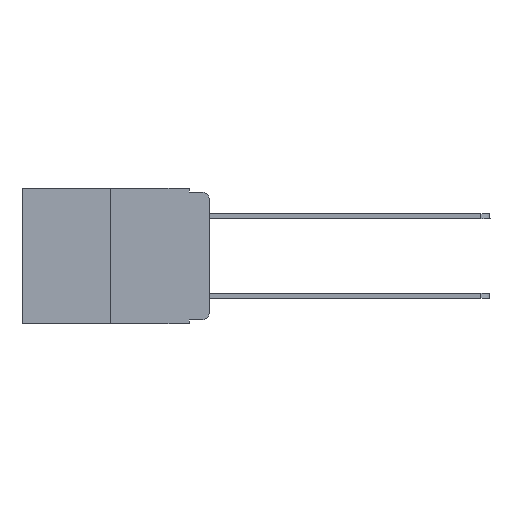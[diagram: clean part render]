
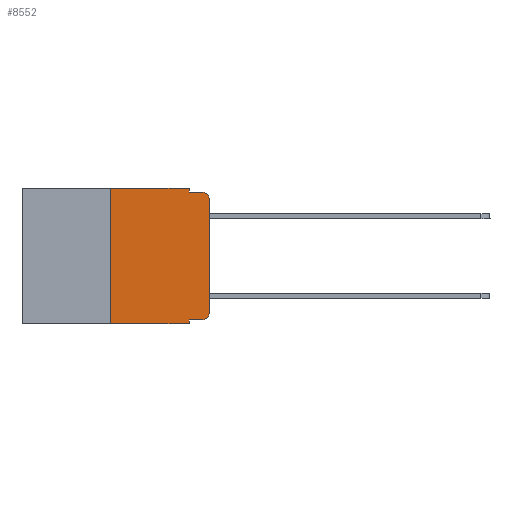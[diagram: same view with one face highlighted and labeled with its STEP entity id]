
A CAD part, left-side view. The second image highlights one B-rep face of the part: STEP entity #8552.
In plain terms, the highlighted planar face has unit normal (-1, 0, 0).
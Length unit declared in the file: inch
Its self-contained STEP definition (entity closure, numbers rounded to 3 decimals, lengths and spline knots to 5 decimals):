
#373 = VERTEX_POINT ( 'NONE', #17408 ) ;
#521 = CARTESIAN_POINT ( 'NONE',  ( 0., 0.473, 0. ) ) ;
#603 = EDGE_CURVE ( 'NONE', #18693, #10837, #5304, .T. ) ;
#614 = AXIS2_PLACEMENT_3D ( 'NONE', #3206, #13170, #5791 ) ;
#1064 = CARTESIAN_POINT ( 'NONE',  ( 0., 0.051, -0.333 ) ) ;
#1275 = EDGE_CURVE ( 'NONE', #373, #6326, #12994, .T. ) ;
#1314 = VERTEX_POINT ( 'NONE', #6936 ) ;
#2225 = DIRECTION ( 'NONE',  ( 0., 0., -1. ) ) ;
#2243 = CARTESIAN_POINT ( 'NONE',  ( 0., 0.051, -0.333 ) ) ;
#2625 = DIRECTION ( 'NONE',  ( 0., 0., 1. ) ) ;
#2701 = PLANE ( 'NONE',  #10862 ) ;
#3132 = DIRECTION ( 'NONE',  ( 0., 0., -1. ) ) ;
#3206 = CARTESIAN_POINT ( 'NONE',  ( 0., 0.02, -0.03 ) ) ;
#3434 = ORIENTED_EDGE ( 'NONE', *, *, #9891, .T. ) ;
#3514 = DIRECTION ( 'NONE',  ( 0., 0., 1. ) ) ;
#3793 = LINE ( 'NONE', #13692, #14360 ) ;
#3871 = ORIENTED_EDGE ( 'NONE', *, *, #7501, .F. ) ;
#4732 = ORIENTED_EDGE ( 'NONE', *, *, #14729, .F. ) ;
#4802 = VERTEX_POINT ( 'NONE', #12134 ) ;
#5304 = LINE ( 'NONE', #2243, #15109 ) ;
#5512 = CARTESIAN_POINT ( 'NONE',  ( 0., 0., 0. ) ) ;
#5516 = CARTESIAN_POINT ( 'NONE',  ( 0., 0.473, -0.343 ) ) ;
#5690 = VECTOR ( 'NONE', #13090, 39.37008 ) ;
#5791 = DIRECTION ( 'NONE',  ( 0., 0., -1. ) ) ;
#5926 = VECTOR ( 'NONE', #16604, 39.37008 ) ;
#6326 = VERTEX_POINT ( 'NONE', #17618 ) ;
#6330 = CARTESIAN_POINT ( 'NONE',  ( 0., 0.051, 0. ) ) ;
#6529 = EDGE_CURVE ( 'NONE', #18693, #12720, #14826, .T. ) ;
#6668 = LINE ( 'NONE', #16842, #16408 ) ;
#6718 = DIRECTION ( 'NONE',  ( -1., 0., 0. ) ) ;
#6936 = CARTESIAN_POINT ( 'NONE',  ( 0., 0.25, -0.343 ) ) ;
#7199 = DIRECTION ( 'NONE',  ( 0., 0., -1. ) ) ;
#7232 = LINE ( 'NONE', #5516, #5690 ) ;
#7285 = CARTESIAN_POINT ( 'NONE',  ( 0., 0.02, -0.333 ) ) ;
#7501 = EDGE_CURVE ( 'NONE', #4802, #18412, #10755, .T. ) ;
#8092 = DIRECTION ( 'NONE',  ( 0., -1., 0. ) ) ;
#8180 = VERTEX_POINT ( 'NONE', #17965 ) ;
#8224 = VECTOR ( 'NONE', #9447, 39.37008 ) ;
#8261 = CARTESIAN_POINT ( 'NONE',  ( 0., 0.02, -0.313 ) ) ;
#8552 = ADVANCED_FACE ( 'NONE', ( #10100 ), #2701, .F. ) ;
#9447 = DIRECTION ( 'NONE',  ( 0., -1., 0. ) ) ;
#9670 = VECTOR ( 'NONE', #3132, 39.37008 ) ;
#9709 = EDGE_CURVE ( 'NONE', #1314, #18330, #6668, .T. ) ;
#9891 = EDGE_CURVE ( 'NONE', #1314, #12720, #7232, .T. ) ;
#10100 = FACE_OUTER_BOUND ( 'NONE', #14731, .T. ) ;
#10689 = CARTESIAN_POINT ( 'NONE',  ( 0., 0.051, -0.01 ) ) ;
#10755 = LINE ( 'NONE', #6330, #5926 ) ;
#10837 = VERTEX_POINT ( 'NONE', #7285 ) ;
#10862 = AXIS2_PLACEMENT_3D ( 'NONE', #17279, #13059, #7199 ) ;
#11073 = LINE ( 'NONE', #521, #8224 ) ;
#11777 = CARTESIAN_POINT ( 'NONE',  ( 0., 0.051, -0.343 ) ) ;
#12031 = VECTOR ( 'NONE', #2625, 39.37008 ) ;
#12134 = CARTESIAN_POINT ( 'NONE',  ( 0., 0.051, 0. ) ) ;
#12140 = CARTESIAN_POINT ( 'NONE',  ( 0., 0.051, 0. ) ) ;
#12720 = VERTEX_POINT ( 'NONE', #11777 ) ;
#12777 = CIRCLE ( 'NONE', #14914, 0.02 ) ;
#12886 = ORIENTED_EDGE ( 'NONE', *, *, #603, .T. ) ;
#12988 = CARTESIAN_POINT ( 'NONE',  ( 0., 0.25, 0. ) ) ;
#12994 = LINE ( 'NONE', #5512, #12031 ) ;
#13059 = DIRECTION ( 'NONE',  ( 1., 0., 0. ) ) ;
#13090 = DIRECTION ( 'NONE',  ( 0., -1., 0. ) ) ;
#13170 = DIRECTION ( 'NONE',  ( -1., 0., 0. ) ) ;
#13251 = EDGE_CURVE ( 'NONE', #10837, #373, #12777, .T. ) ;
#13519 = ORIENTED_EDGE ( 'NONE', *, *, #16410, .T. ) ;
#13692 = CARTESIAN_POINT ( 'NONE',  ( 0., 0.051, -0.01 ) ) ;
#13977 = ORIENTED_EDGE ( 'NONE', *, *, #13251, .T. ) ;
#14360 = VECTOR ( 'NONE', #18377, 39.37008 ) ;
#14369 = EDGE_CURVE ( 'NONE', #18412, #8180, #3793, .T. ) ;
#14729 = EDGE_CURVE ( 'NONE', #18330, #4802, #11073, .T. ) ;
#14731 = EDGE_LOOP ( 'NONE', ( #15907, #13519, #16361, #3871, #4732, #17921, #3434, #16491, #12886, #13977 ) ) ;
#14826 = LINE ( 'NONE', #12140, #9670 ) ;
#14914 = AXIS2_PLACEMENT_3D ( 'NONE', #8261, #6718, #2225 ) ;
#15109 = VECTOR ( 'NONE', #8092, 39.37008 ) ;
#15907 = ORIENTED_EDGE ( 'NONE', *, *, #1275, .T. ) ;
#16361 = ORIENTED_EDGE ( 'NONE', *, *, #14369, .F. ) ;
#16408 = VECTOR ( 'NONE', #3514, 39.37008 ) ;
#16410 = EDGE_CURVE ( 'NONE', #6326, #8180, #17480, .T. ) ;
#16491 = ORIENTED_EDGE ( 'NONE', *, *, #6529, .F. ) ;
#16604 = DIRECTION ( 'NONE',  ( 0., 0., -1. ) ) ;
#16842 = CARTESIAN_POINT ( 'NONE',  ( 0., 0.25, 0. ) ) ;
#17279 = CARTESIAN_POINT ( 'NONE',  ( 0., 0.473, 0. ) ) ;
#17408 = CARTESIAN_POINT ( 'NONE',  ( 0., 0., -0.313 ) ) ;
#17480 = CIRCLE ( 'NONE', #614, 0.02 ) ;
#17618 = CARTESIAN_POINT ( 'NONE',  ( 0., 0., -0.03 ) ) ;
#17921 = ORIENTED_EDGE ( 'NONE', *, *, #9709, .F. ) ;
#17965 = CARTESIAN_POINT ( 'NONE',  ( 0., 0.02, -0.01 ) ) ;
#18330 = VERTEX_POINT ( 'NONE', #12988 ) ;
#18377 = DIRECTION ( 'NONE',  ( 0., -1., 0. ) ) ;
#18412 = VERTEX_POINT ( 'NONE', #10689 ) ;
#18693 = VERTEX_POINT ( 'NONE', #1064 ) ;
